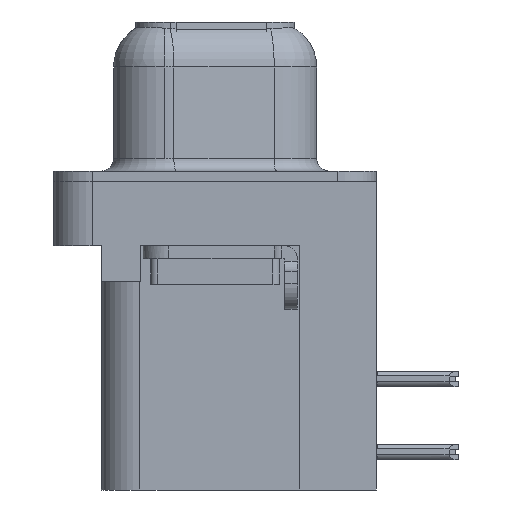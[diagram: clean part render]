
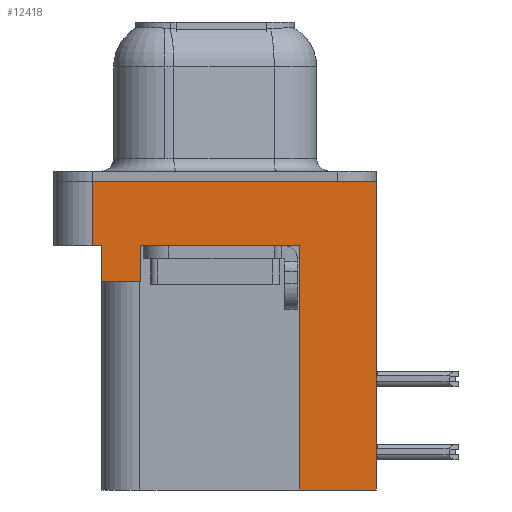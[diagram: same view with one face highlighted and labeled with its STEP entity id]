
A CAD part, left-side view. The second image highlights one B-rep face of the part: STEP entity #12418.
In plain terms, the highlighted planar face has unit normal (-1, 0, 0).
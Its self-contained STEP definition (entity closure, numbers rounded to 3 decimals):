
#182 = VECTOR ( 'NONE', #15565, 1000. ) ;
#187 = LINE ( 'NONE', #13915, #21405 ) ;
#615 = EDGE_CURVE ( 'NONE', #22386, #11388, #15854, .T. ) ;
#700 = LINE ( 'NONE', #11476, #21950 ) ;
#902 = FACE_OUTER_BOUND ( 'NONE', #23831, .T. ) ;
#1332 = ORIENTED_EDGE ( 'NONE', *, *, #17168, .F. ) ;
#1691 = CARTESIAN_POINT ( 'NONE',  ( -2.935, 4.775, -2.5 ) ) ;
#1855 = VERTEX_POINT ( 'NONE', #5590 ) ;
#1991 = PLANE ( 'NONE',  #13118 ) ;
#2088 = CARTESIAN_POINT ( 'NONE',  ( -2.935, -6.275, -2.5 ) ) ;
#2185 = LINE ( 'NONE', #9422, #22733 ) ;
#2313 = ORIENTED_EDGE ( 'NONE', *, *, #17321, .T. ) ;
#2511 = LINE ( 'NONE', #1691, #23661 ) ;
#2694 = VECTOR ( 'NONE', #14920, 1000. ) ;
#2986 = CARTESIAN_POINT ( 'NONE',  ( -2.935, -6.275, 0. ) ) ;
#3238 = DIRECTION ( 'NONE',  ( 0., 0., 1. ) ) ;
#3417 = ORIENTED_EDGE ( 'NONE', *, *, #12734, .F. ) ;
#3772 = VERTEX_POINT ( 'NONE', #15170 ) ;
#3847 = VERTEX_POINT ( 'NONE', #23623 ) ;
#4236 = DIRECTION ( 'NONE',  ( 0., 0., 1. ) ) ;
#4357 = ORIENTED_EDGE ( 'NONE', *, *, #26387, .F. ) ;
#5590 = CARTESIAN_POINT ( 'NONE',  ( -2.935, 2.895, -3.9 ) ) ;
#5798 = DIRECTION ( 'NONE',  ( 0., -1., 0. ) ) ;
#5875 = EDGE_CURVE ( 'NONE', #9461, #3772, #14693, .T. ) ;
#5965 = DIRECTION ( 'NONE',  ( 0., 0., 1. ) ) ;
#6003 = VECTOR ( 'NONE', #5965, 1000. ) ;
#6684 = LINE ( 'NONE', #16132, #6003 ) ;
#6876 = VECTOR ( 'NONE', #9062, 1000. ) ;
#7265 = EDGE_CURVE ( 'NONE', #3772, #3847, #6684, .T. ) ;
#7656 = VERTEX_POINT ( 'NONE', #19291 ) ;
#7755 = ORIENTED_EDGE ( 'NONE', *, *, #24040, .F. ) ;
#7892 = DIRECTION ( 'NONE',  ( 0., 0., 1. ) ) ;
#7978 = ORIENTED_EDGE ( 'NONE', *, *, #13426, .T. ) ;
#8138 = VERTEX_POINT ( 'NONE', #22992 ) ;
#9012 = VERTEX_POINT ( 'NONE', #22596 ) ;
#9062 = DIRECTION ( 'NONE',  ( 0., -1., 0. ) ) ;
#9064 = CARTESIAN_POINT ( 'NONE',  ( -2.935, -6.275, -2.5 ) ) ;
#9422 = CARTESIAN_POINT ( 'NONE',  ( -2.935, 4.425, -3.9 ) ) ;
#9461 = VERTEX_POINT ( 'NONE', #11792 ) ;
#9889 = VERTEX_POINT ( 'NONE', #21565 ) ;
#11127 = VECTOR ( 'NONE', #5798, 1000. ) ;
#11388 = VERTEX_POINT ( 'NONE', #24838 ) ;
#11476 = CARTESIAN_POINT ( 'NONE',  ( -2.935, -6.275, -2.5 ) ) ;
#11792 = CARTESIAN_POINT ( 'NONE',  ( -2.935, -6.275, -12. ) ) ;
#12189 = ORIENTED_EDGE ( 'NONE', *, *, #26557, .T. ) ;
#12418 = ADVANCED_FACE ( 'NONE', ( #902 ), #1991, .T. ) ;
#12734 = EDGE_CURVE ( 'NONE', #9012, #11388, #2185, .T. ) ;
#13118 = AXIS2_PLACEMENT_3D ( 'NONE', #2088, #16452, #4236 ) ;
#13426 = EDGE_CURVE ( 'NONE', #1855, #8138, #187, .T. ) ;
#13507 = CARTESIAN_POINT ( 'NONE',  ( -2.935, -3.295, -12. ) ) ;
#13642 = LINE ( 'NONE', #25183, #2694 ) ;
#13915 = CARTESIAN_POINT ( 'NONE',  ( -2.935, 2.895, -3.9 ) ) ;
#14042 = DIRECTION ( 'NONE',  ( 0., 0., 1. ) ) ;
#14693 = LINE ( 'NONE', #13507, #182 ) ;
#14920 = DIRECTION ( 'NONE',  ( 0., 1., 0. ) ) ;
#15170 = CARTESIAN_POINT ( 'NONE',  ( -2.935, -3.295, -12. ) ) ;
#15565 = DIRECTION ( 'NONE',  ( 0., 1., 0. ) ) ;
#15854 = LINE ( 'NONE', #24138, #11127 ) ;
#16132 = CARTESIAN_POINT ( 'NONE',  ( -2.935, -3.295, -12. ) ) ;
#16452 = DIRECTION ( 'NONE',  ( -1., 0., 0. ) ) ;
#17168 = EDGE_CURVE ( 'NONE', #1855, #9012, #13642, .T. ) ;
#17321 = EDGE_CURVE ( 'NONE', #9461, #9889, #700, .T. ) ;
#19291 = CARTESIAN_POINT ( 'NONE',  ( -2.935, 4.775, 0. ) ) ;
#19832 = ORIENTED_EDGE ( 'NONE', *, *, #615, .T. ) ;
#20460 = LINE ( 'NONE', #9064, #26493 ) ;
#21405 = VECTOR ( 'NONE', #7892, 1000. ) ;
#21565 = CARTESIAN_POINT ( 'NONE',  ( -2.935, -6.275, 0. ) ) ;
#21950 = VECTOR ( 'NONE', #3238, 1000. ) ;
#22386 = VERTEX_POINT ( 'NONE', #26505 ) ;
#22514 = LINE ( 'NONE', #2986, #6876 ) ;
#22596 = CARTESIAN_POINT ( 'NONE',  ( -2.935, 4.425, -3.9 ) ) ;
#22733 = VECTOR ( 'NONE', #23675, 1000. ) ;
#22992 = CARTESIAN_POINT ( 'NONE',  ( -2.935, 2.895, -2.5 ) ) ;
#23327 = DIRECTION ( 'NONE',  ( 0., -1., 0. ) ) ;
#23623 = CARTESIAN_POINT ( 'NONE',  ( -2.935, -3.295, -2.5 ) ) ;
#23651 = ORIENTED_EDGE ( 'NONE', *, *, #5875, .F. ) ;
#23661 = VECTOR ( 'NONE', #14042, 1000. ) ;
#23675 = DIRECTION ( 'NONE',  ( 0., 0., 1. ) ) ;
#23831 = EDGE_LOOP ( 'NONE', ( #7755, #4357, #19832, #3417, #1332, #7978, #12189, #26085, #23651, #2313 ) ) ;
#24040 = EDGE_CURVE ( 'NONE', #7656, #9889, #22514, .T. ) ;
#24138 = CARTESIAN_POINT ( 'NONE',  ( -2.935, -6.275, -2.5 ) ) ;
#24838 = CARTESIAN_POINT ( 'NONE',  ( -2.935, 4.425, -2.5 ) ) ;
#25183 = CARTESIAN_POINT ( 'NONE',  ( -2.935, 4.425, -3.9 ) ) ;
#26085 = ORIENTED_EDGE ( 'NONE', *, *, #7265, .F. ) ;
#26387 = EDGE_CURVE ( 'NONE', #22386, #7656, #2511, .T. ) ;
#26493 = VECTOR ( 'NONE', #23327, 1000. ) ;
#26505 = CARTESIAN_POINT ( 'NONE',  ( -2.935, 4.775, -2.5 ) ) ;
#26557 = EDGE_CURVE ( 'NONE', #8138, #3847, #20460, .T. ) ;
